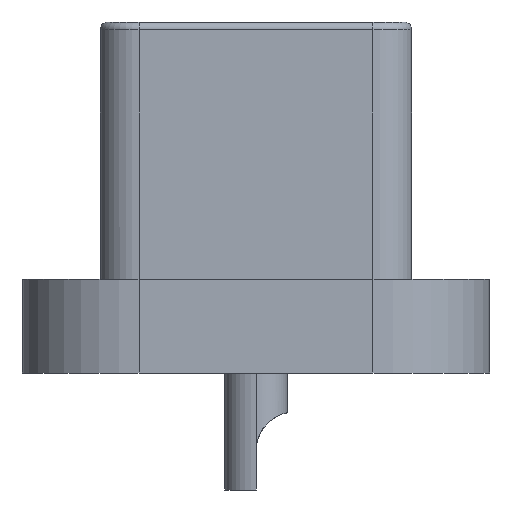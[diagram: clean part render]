
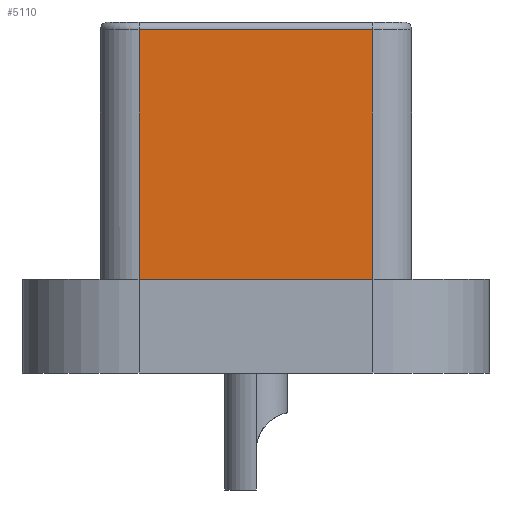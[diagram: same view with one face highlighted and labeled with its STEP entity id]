
A CAD part, left-side view. The second image highlights one B-rep face of the part: STEP entity #5110.
In plain terms, the highlighted planar face has unit normal (-1, 0, 0).
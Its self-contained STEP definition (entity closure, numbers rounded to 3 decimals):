
#492 = ORIENTED_EDGE ( 'NONE', *, *, #6283, .T. ) ;
#519 = CARTESIAN_POINT ( 'NONE',  ( -8.45, 1.5, -3.3 ) ) ;
#524 = DIRECTION ( 'NONE',  ( 0., 1., 0. ) ) ;
#582 = CARTESIAN_POINT ( 'NONE',  ( -8.45, -1.5, -0.1 ) ) ;
#914 = LINE ( 'NONE', #3210, #5897 ) ;
#930 = VECTOR ( 'NONE', #2787, 1000. ) ;
#1074 = PLANE ( 'NONE',  #4353 ) ;
#1225 = ORIENTED_EDGE ( 'NONE', *, *, #3813, .T. ) ;
#1541 = DIRECTION ( 'NONE',  ( 0., 0., 1. ) ) ;
#2754 = VERTEX_POINT ( 'NONE', #6085 ) ;
#2787 = DIRECTION ( 'NONE',  ( 0., -1., 0. ) ) ;
#2841 = DIRECTION ( 'NONE',  ( 0., 1., 0. ) ) ;
#3118 = EDGE_LOOP ( 'NONE', ( #4455, #5315, #1225, #492 ) ) ;
#3171 = VERTEX_POINT ( 'NONE', #5106 ) ;
#3210 = CARTESIAN_POINT ( 'NONE',  ( -8.45, 1.5, -0.1 ) ) ;
#3293 = CARTESIAN_POINT ( 'NONE',  ( -8.45, 1.5, -3.3 ) ) ;
#3380 = EDGE_CURVE ( 'NONE', #4627, #6166, #914, .T. ) ;
#3389 = CARTESIAN_POINT ( 'NONE',  ( -8.45, 0., -1.7 ) ) ;
#3813 = EDGE_CURVE ( 'NONE', #3171, #2754, #4442, .T. ) ;
#4353 = AXIS2_PLACEMENT_3D ( 'NONE', #3389, #5733, #524 ) ;
#4442 = LINE ( 'NONE', #6757, #4528 ) ;
#4455 = ORIENTED_EDGE ( 'NONE', *, *, #3380, .T. ) ;
#4528 = VECTOR ( 'NONE', #1541, 1000. ) ;
#4627 = VERTEX_POINT ( 'NONE', #5914 ) ;
#5106 = CARTESIAN_POINT ( 'NONE',  ( -8.45, -1.5, -3.3 ) ) ;
#5110 = ADVANCED_FACE ( 'NONE', ( #6305 ), #1074, .F. ) ;
#5315 = ORIENTED_EDGE ( 'NONE', *, *, #6842, .T. ) ;
#5434 = VECTOR ( 'NONE', #2841, 1000. ) ;
#5548 = DIRECTION ( 'NONE',  ( 0., 0., -1. ) ) ;
#5726 = LINE ( 'NONE', #519, #930 ) ;
#5733 = DIRECTION ( 'NONE',  ( 1., 0., 0. ) ) ;
#5779 = LINE ( 'NONE', #582, #5434 ) ;
#5897 = VECTOR ( 'NONE', #5548, 1000. ) ;
#5914 = CARTESIAN_POINT ( 'NONE',  ( -8.45, 1.5, -0.1 ) ) ;
#6085 = CARTESIAN_POINT ( 'NONE',  ( -8.45, -1.5, -0.1 ) ) ;
#6166 = VERTEX_POINT ( 'NONE', #3293 ) ;
#6283 = EDGE_CURVE ( 'NONE', #2754, #4627, #5779, .T. ) ;
#6305 = FACE_OUTER_BOUND ( 'NONE', #3118, .T. ) ;
#6757 = CARTESIAN_POINT ( 'NONE',  ( -8.45, -1.5, -3.3 ) ) ;
#6842 = EDGE_CURVE ( 'NONE', #6166, #3171, #5726, .T. ) ;
